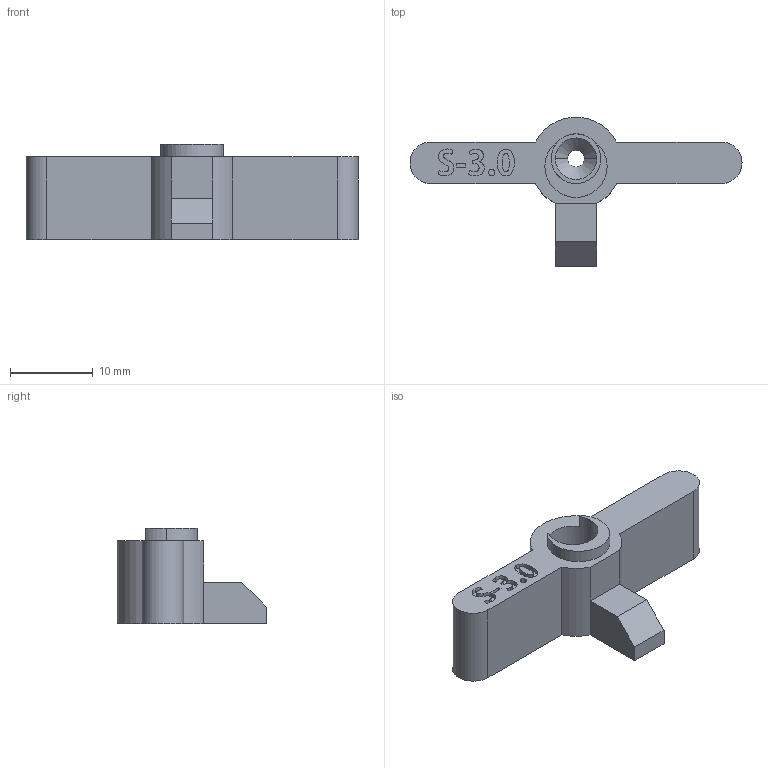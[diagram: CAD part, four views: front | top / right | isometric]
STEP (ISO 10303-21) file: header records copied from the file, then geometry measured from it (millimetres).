
FILE_DESCRIPTION (( 'STEP AP214' ), '1' );
FILE_NAME ('Bolt^StikM1.STEP', '2013-09-01T22:38:51', ( 'Asher' ), ( '' ), 'SwSTEP 2.0', 'SolidWorks 2013', '' );
FILE_SCHEMA (( 'AUTOMOTIVE_DESIGN' ));
Length unit declared in the file: millimetre
Products named in the file (1): Bolt^StikM1
Bounding box: 40 x 17.98 x 11.5 mm (x, y, z)
Volume: 2364.2 mm3; surface area: 1691 mm2
Topology: 1 solids, 1 shells, 92 faces, 245 edges, 162 vertices
Faces by surface type: bspline 36, plane 35, cylinder 19, cone 2
Entity records: 4812 total; most frequent: CARTESIAN_POINT 2700, ORIENTED_EDGE 490, DIRECTION 320, EDGE_CURVE 245, VERTEX_POINT 162, LINE 132, VECTOR 132, EDGE_LOOP 101
